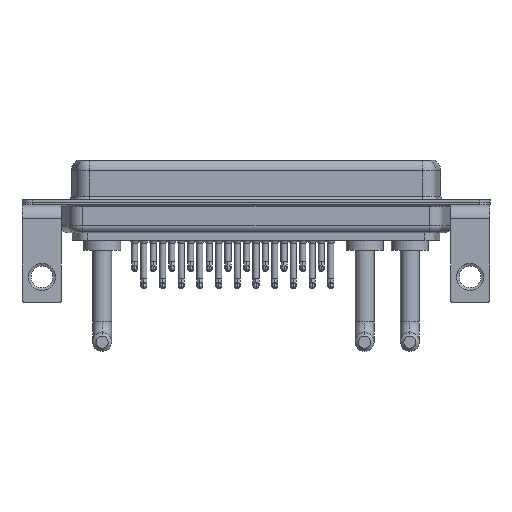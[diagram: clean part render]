
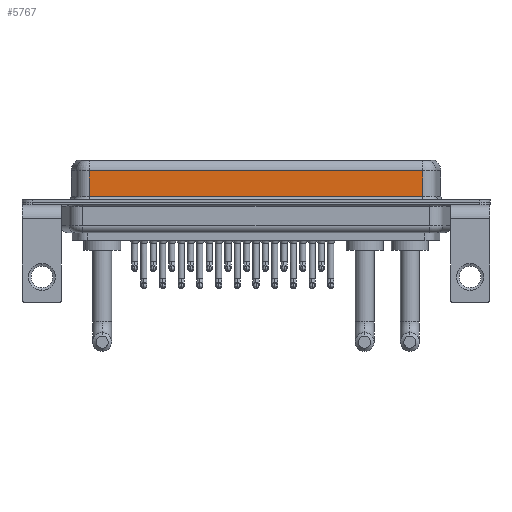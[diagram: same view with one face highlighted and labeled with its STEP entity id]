
A CAD part, front view. The second image highlights one B-rep face of the part: STEP entity #5767.
In plain terms, the highlighted planar face has unit normal (0, -1, 0).
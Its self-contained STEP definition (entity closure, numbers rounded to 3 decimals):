
#844 = VECTOR ( 'NONE', #17134, 1000. ) ;
#2370 = DIRECTION ( 'NONE',  ( 0., 0., -1. ) ) ;
#4810 = VERTEX_POINT ( 'NONE', #19809 ) ;
#4925 = CARTESIAN_POINT ( 'NONE',  ( 56.462, -3.95, 4.65 ) ) ;
#5339 = FACE_OUTER_BOUND ( 'NONE', #16960, .T. ) ;
#5712 = DIRECTION ( 'NONE',  ( 0., 0., 1. ) ) ;
#5767 = ADVANCED_FACE ( 'NONE', ( #5339 ), #9310, .F. ) ;
#7552 = CARTESIAN_POINT ( 'NONE',  ( 56.462, -3.95, 6.4 ) ) ;
#7741 = CARTESIAN_POINT ( 'NONE',  ( 7.038, -3.95, 6.4 ) ) ;
#8048 = VECTOR ( 'NONE', #19669, 1000. ) ;
#9279 = VERTEX_POINT ( 'NONE', #12632 ) ;
#9310 = PLANE ( 'NONE',  #16642 ) ;
#9797 = VERTEX_POINT ( 'NONE', #16409 ) ;
#10278 = CARTESIAN_POINT ( 'NONE',  ( 56.462, -3.95, 0.9 ) ) ;
#11911 = VERTEX_POINT ( 'NONE', #19501 ) ;
#12632 = CARTESIAN_POINT ( 'NONE',  ( 7.038, -3.95, 0.9 ) ) ;
#12688 = ORIENTED_EDGE ( 'NONE', *, *, #13217, .F. ) ;
#13217 = EDGE_CURVE ( 'NONE', #11911, #9797, #20757, .T. ) ;
#13817 = LINE ( 'NONE', #4925, #8048 ) ;
#14030 = EDGE_CURVE ( 'NONE', #9279, #9797, #18133, .T. ) ;
#16409 = CARTESIAN_POINT ( 'NONE',  ( 56.462, -3.95, 0.9 ) ) ;
#16642 = AXIS2_PLACEMENT_3D ( 'NONE', #22631, #18668, #5712 ) ;
#16960 = EDGE_LOOP ( 'NONE', ( #12688, #23609, #20226, #23239 ) ) ;
#17134 = DIRECTION ( 'NONE',  ( 0., 0., -1. ) ) ;
#17287 = EDGE_CURVE ( 'NONE', #4810, #9279, #21540, .T. ) ;
#18133 = LINE ( 'NONE', #10278, #20765 ) ;
#18668 = DIRECTION ( 'NONE',  ( 0., 1., 0. ) ) ;
#19501 = CARTESIAN_POINT ( 'NONE',  ( 56.462, -3.95, 4.65 ) ) ;
#19669 = DIRECTION ( 'NONE',  ( -1., 0., 0. ) ) ;
#19809 = CARTESIAN_POINT ( 'NONE',  ( 7.038, -3.95, 4.65 ) ) ;
#19988 = DIRECTION ( 'NONE',  ( 1., 0., 0. ) ) ;
#20226 = ORIENTED_EDGE ( 'NONE', *, *, #17287, .T. ) ;
#20757 = LINE ( 'NONE', #7552, #844 ) ;
#20765 = VECTOR ( 'NONE', #19988, 1000. ) ;
#21540 = LINE ( 'NONE', #7741, #24013 ) ;
#22631 = CARTESIAN_POINT ( 'NONE',  ( 56.462, -3.95, 6.4 ) ) ;
#23229 = EDGE_CURVE ( 'NONE', #11911, #4810, #13817, .T. ) ;
#23239 = ORIENTED_EDGE ( 'NONE', *, *, #14030, .T. ) ;
#23609 = ORIENTED_EDGE ( 'NONE', *, *, #23229, .T. ) ;
#24013 = VECTOR ( 'NONE', #2370, 1000. ) ;
